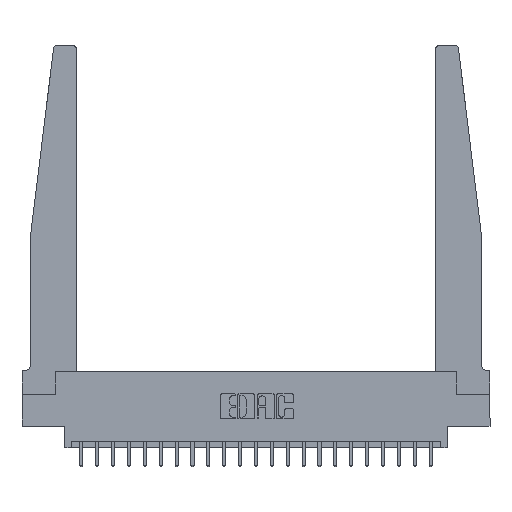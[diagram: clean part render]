
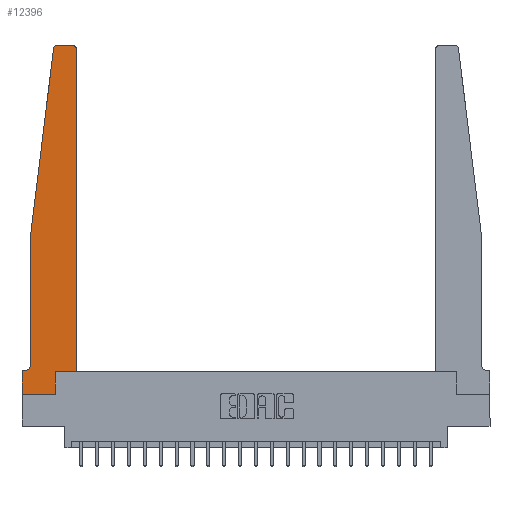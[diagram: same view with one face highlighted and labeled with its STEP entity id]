
A CAD part, top view. The second image highlights one B-rep face of the part: STEP entity #12396.
In plain terms, the highlighted planar face has unit normal (0, 0, 1).
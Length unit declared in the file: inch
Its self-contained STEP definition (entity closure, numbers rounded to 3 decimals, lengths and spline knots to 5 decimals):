
#31 = EDGE_CURVE ( 'NONE', #19976, #5698, #18367, .T. ) ;
#395 = VERTEX_POINT ( 'NONE', #17955 ) ;
#459 = VERTEX_POINT ( 'NONE', #21475 ) ;
#629 = CARTESIAN_POINT ( 'NONE',  ( 0.27653, 2.75, 0.37 ) ) ;
#761 = DIRECTION ( 'NONE',  ( 1., 0., 0. ) ) ;
#781 = ORIENTED_EDGE ( 'NONE', *, *, #22292, .T. ) ;
#1077 = CARTESIAN_POINT ( 'NONE',  ( 0.395, 2.72, 0.37 ) ) ;
#1081 = ORIENTED_EDGE ( 'NONE', *, *, #21896, .T. ) ;
#1175 = ORIENTED_EDGE ( 'NONE', *, *, #31, .T. ) ;
#1683 = CARTESIAN_POINT ( 'NONE',  ( 0.2605, 0., 0.37 ) ) ;
#1816 = DIRECTION ( 'NONE',  ( 0., 1., 0. ) ) ;
#1825 = CARTESIAN_POINT ( 'NONE',  ( 0., 0.1875, 0.37 ) ) ;
#1828 = DIRECTION ( 'NONE',  ( -0.122, -0.992, 0. ) ) ;
#2192 = ORIENTED_EDGE ( 'NONE', *, *, #16532, .T. ) ;
#2210 = ORIENTED_EDGE ( 'NONE', *, *, #7381, .T. ) ;
#2446 = ORIENTED_EDGE ( 'NONE', *, *, #2628, .T. ) ;
#2628 = EDGE_CURVE ( 'NONE', #12875, #15649, #13468, .T. ) ;
#2798 = CIRCLE ( 'NONE', #10481, 0.03 ) ;
#2872 = DIRECTION ( 'NONE',  ( 1., 0., 0. ) ) ;
#2960 = DIRECTION ( 'NONE',  ( 0., 0., -1. ) ) ;
#3094 = ORIENTED_EDGE ( 'NONE', *, *, #17147, .T. ) ;
#3181 = CARTESIAN_POINT ( 'NONE',  ( 0.065, 1.25, 0.37 ) ) ;
#3631 = VECTOR ( 'NONE', #16908, 39.37008 ) ;
#3693 = LINE ( 'NONE', #20955, #17126 ) ;
#3772 = DIRECTION ( 'NONE',  ( 0., 1., 0. ) ) ;
#3903 = CARTESIAN_POINT ( 'NONE',  ( 0.425, 2.72, 0.37 ) ) ;
#4706 = CARTESIAN_POINT ( 'NONE',  ( 0.25, 2.75, 0.37 ) ) ;
#4820 = LINE ( 'NONE', #12979, #13113 ) ;
#4829 = LINE ( 'NONE', #14678, #17617 ) ;
#5046 = EDGE_CURVE ( 'NONE', #15649, #20385, #3693, .T. ) ;
#5181 = DIRECTION ( 'NONE',  ( 1., 0., 0. ) ) ;
#5414 = CARTESIAN_POINT ( 'NONE',  ( 0.27653, 2.72, 0.37 ) ) ;
#5452 = DIRECTION ( 'NONE',  ( 1., 0., 0. ) ) ;
#5494 = EDGE_CURVE ( 'NONE', #20135, #19976, #4829, .T. ) ;
#5698 = VERTEX_POINT ( 'NONE', #10021 ) ;
#6059 = CARTESIAN_POINT ( 'NONE',  ( 0.065, 0.1875, 0.37 ) ) ;
#6456 = VECTOR ( 'NONE', #1828, 39.37008 ) ;
#7042 = VECTOR ( 'NONE', #7816, 39.37008 ) ;
#7196 = DIRECTION ( 'NONE',  ( 1., 0., 0. ) ) ;
#7212 = VECTOR ( 'NONE', #5181, 39.37008 ) ;
#7381 = EDGE_CURVE ( 'NONE', #7837, #12875, #9850, .T. ) ;
#7421 = CARTESIAN_POINT ( 'NONE',  ( 0.2605, 0.18, 0.37 ) ) ;
#7686 = VERTEX_POINT ( 'NONE', #16853 ) ;
#7816 = DIRECTION ( 'NONE',  ( -1., 0., 0. ) ) ;
#7837 = VERTEX_POINT ( 'NONE', #1683 ) ;
#7842 = LINE ( 'NONE', #4706, #3631 ) ;
#7906 = PLANE ( 'NONE',  #8329 ) ;
#8329 = AXIS2_PLACEMENT_3D ( 'NONE', #13143, #11463, #761 ) ;
#8336 = AXIS2_PLACEMENT_3D ( 'NONE', #13618, #2960, #15346 ) ;
#8592 = EDGE_LOOP ( 'NONE', ( #781, #13184, #1081, #13422, #1175, #13596, #2192, #13729, #2210, #2446, #13931, #3094 ) ) ;
#8930 = CARTESIAN_POINT ( 'NONE',  ( 0.425, 0.18, 0.37 ) ) ;
#9850 = LINE ( 'NONE', #16061, #17890 ) ;
#10021 = CARTESIAN_POINT ( 'NONE',  ( 0.015, 0.1875, 0.37 ) ) ;
#10225 = VERTEX_POINT ( 'NONE', #1825 ) ;
#10481 = AXIS2_PLACEMENT_3D ( 'NONE', #1077, #13531, #2872 ) ;
#10806 = EDGE_CURVE ( 'NONE', #459, #7837, #19874, .T. ) ;
#11153 = LINE ( 'NONE', #19300, #6456 ) ;
#11463 = DIRECTION ( 'NONE',  ( 0., 0., 1. ) ) ;
#12327 = CARTESIAN_POINT ( 'NONE',  ( 0.425, 0.18, 0.37 ) ) ;
#12396 = ADVANCED_FACE ( 'NONE', ( #17987 ), #7906, .T. ) ;
#12875 = VERTEX_POINT ( 'NONE', #7421 ) ;
#12979 = CARTESIAN_POINT ( 'NONE',  ( 0., 0., 0.37 ) ) ;
#13113 = VECTOR ( 'NONE', #14714, 39.37008 ) ;
#13143 = CARTESIAN_POINT ( 'NONE',  ( 0., 0.1875, 0.37 ) ) ;
#13184 = ORIENTED_EDGE ( 'NONE', *, *, #20904, .T. ) ;
#13422 = ORIENTED_EDGE ( 'NONE', *, *, #5494, .T. ) ;
#13468 = LINE ( 'NONE', #8930, #16920 ) ;
#13531 = DIRECTION ( 'NONE',  ( 0., 0., 1. ) ) ;
#13596 = ORIENTED_EDGE ( 'NONE', *, *, #22125, .T. ) ;
#13618 = CARTESIAN_POINT ( 'NONE',  ( 0.015, 0.2375, 0.37 ) ) ;
#13729 = ORIENTED_EDGE ( 'NONE', *, *, #10806, .T. ) ;
#13931 = ORIENTED_EDGE ( 'NONE', *, *, #5046, .T. ) ;
#14678 = CARTESIAN_POINT ( 'NONE',  ( 0.065, 1.25, 0.37 ) ) ;
#14714 = DIRECTION ( 'NONE',  ( 0., -1., 0. ) ) ;
#15339 = AXIS2_PLACEMENT_3D ( 'NONE', #5414, #17551, #7196 ) ;
#15346 = DIRECTION ( 'NONE',  ( -1., 0., 0. ) ) ;
#15649 = VERTEX_POINT ( 'NONE', #12327 ) ;
#16061 = CARTESIAN_POINT ( 'NONE',  ( 0.2605, 0.18, 0.37 ) ) ;
#16532 = EDGE_CURVE ( 'NONE', #10225, #459, #4820, .T. ) ;
#16853 = CARTESIAN_POINT ( 'NONE',  ( 0.24675, 2.72367, 0.37 ) ) ;
#16855 = CARTESIAN_POINT ( 'NONE',  ( 0.065, 0.2375, 0.37 ) ) ;
#16908 = DIRECTION ( 'NONE',  ( -1., 0., 0. ) ) ;
#16920 = VECTOR ( 'NONE', #5452, 39.37008 ) ;
#17126 = VECTOR ( 'NONE', #1816, 39.37008 ) ;
#17147 = EDGE_CURVE ( 'NONE', #20385, #395, #2798, .T. ) ;
#17275 = CARTESIAN_POINT ( 'NONE',  ( 0., 0., 0.37 ) ) ;
#17551 = DIRECTION ( 'NONE',  ( 0., 0., 1. ) ) ;
#17617 = VECTOR ( 'NONE', #18050, 39.37008 ) ;
#17890 = VECTOR ( 'NONE', #3772, 39.37008 ) ;
#17955 = CARTESIAN_POINT ( 'NONE',  ( 0.395, 2.75, 0.37 ) ) ;
#17987 = FACE_OUTER_BOUND ( 'NONE', #8592, .T. ) ;
#18050 = DIRECTION ( 'NONE',  ( 0., -1., 0. ) ) ;
#18367 = CIRCLE ( 'NONE', #8336, 0.05 ) ;
#19300 = CARTESIAN_POINT ( 'NONE',  ( 0.065, 1.25, 0.37 ) ) ;
#19874 = LINE ( 'NONE', #17275, #7212 ) ;
#19976 = VERTEX_POINT ( 'NONE', #16855 ) ;
#20135 = VERTEX_POINT ( 'NONE', #3181 ) ;
#20385 = VERTEX_POINT ( 'NONE', #3903 ) ;
#20752 = LINE ( 'NONE', #6059, #7042 ) ;
#20770 = CIRCLE ( 'NONE', #15339, 0.03 ) ;
#20904 = EDGE_CURVE ( 'NONE', #21449, #7686, #20770, .T. ) ;
#20955 = CARTESIAN_POINT ( 'NONE',  ( 0.425, 0.18, 0.37 ) ) ;
#21449 = VERTEX_POINT ( 'NONE', #629 ) ;
#21475 = CARTESIAN_POINT ( 'NONE',  ( 0., 0., 0.37 ) ) ;
#21896 = EDGE_CURVE ( 'NONE', #7686, #20135, #11153, .T. ) ;
#22125 = EDGE_CURVE ( 'NONE', #5698, #10225, #20752, .T. ) ;
#22292 = EDGE_CURVE ( 'NONE', #395, #21449, #7842, .T. ) ;
